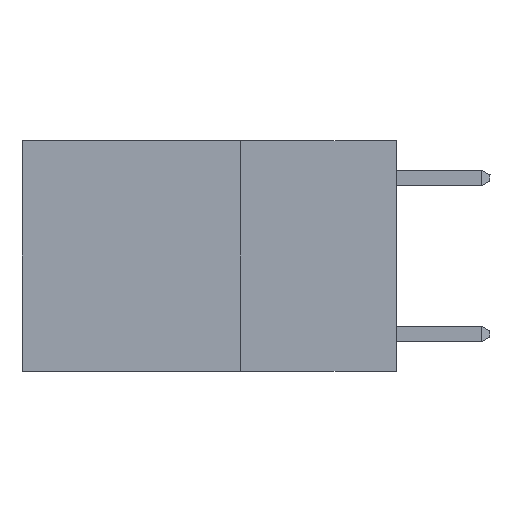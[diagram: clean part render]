
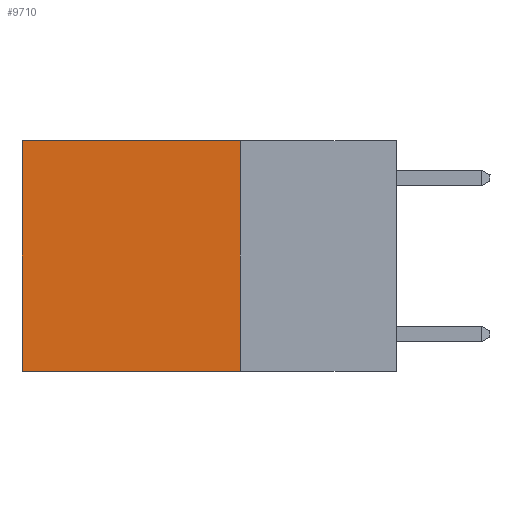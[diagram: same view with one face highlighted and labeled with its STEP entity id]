
A CAD part, left-side view. The second image highlights one B-rep face of the part: STEP entity #9710.
In plain terms, the highlighted planar face has unit normal (-1, 0, 0).
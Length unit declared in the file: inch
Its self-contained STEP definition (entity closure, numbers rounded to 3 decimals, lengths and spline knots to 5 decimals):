
#161 = DIRECTION ( 'NONE',  ( 0., 0., -1. ) ) ;
#735 = PLANE ( 'NONE',  #3707 ) ;
#923 = CARTESIAN_POINT ( 'NONE',  ( 0.2625, 0.6, 0. ) ) ;
#1424 = LINE ( 'NONE', #2410, #9687 ) ;
#2410 = CARTESIAN_POINT ( 'NONE',  ( 0.2625, 0.25, 0. ) ) ;
#3197 = CARTESIAN_POINT ( 'NONE',  ( 0.2625, 0.25, 0. ) ) ;
#3236 = DIRECTION ( 'NONE',  ( 1., 0., 0. ) ) ;
#3293 = ORIENTED_EDGE ( 'NONE', *, *, #4226, .F. ) ;
#3406 = EDGE_CURVE ( 'NONE', #9492, #10022, #1424, .T. ) ;
#3707 = AXIS2_PLACEMENT_3D ( 'NONE', #3197, #3236, #8784 ) ;
#4226 = EDGE_CURVE ( 'NONE', #9492, #7613, #9802, .T. ) ;
#4418 = VERTEX_POINT ( 'NONE', #7597 ) ;
#4994 = ORIENTED_EDGE ( 'NONE', *, *, #3406, .T. ) ;
#5407 = VECTOR ( 'NONE', #161, 39.37008 ) ;
#5448 = ORIENTED_EDGE ( 'NONE', *, *, #9461, .T. ) ;
#5813 = LINE ( 'NONE', #923, #7671 ) ;
#5844 = CARTESIAN_POINT ( 'NONE',  ( 0.2625, 0.25, 0. ) ) ;
#7046 = VECTOR ( 'NONE', #8673, 39.37008 ) ;
#7597 = CARTESIAN_POINT ( 'NONE',  ( 0.2625, 0.6, -0.37 ) ) ;
#7613 = VERTEX_POINT ( 'NONE', #8380 ) ;
#7671 = VECTOR ( 'NONE', #8949, 39.37008 ) ;
#7909 = CARTESIAN_POINT ( 'NONE',  ( 0.2625, 0.25, -0.37 ) ) ;
#8245 = CARTESIAN_POINT ( 'NONE',  ( 0.2625, 0.25, 0. ) ) ;
#8380 = CARTESIAN_POINT ( 'NONE',  ( 0.2625, 0.25, -0.37 ) ) ;
#8398 = FACE_OUTER_BOUND ( 'NONE', #9883, .T. ) ;
#8673 = DIRECTION ( 'NONE',  ( 0., 1., 0. ) ) ;
#8784 = DIRECTION ( 'NONE',  ( 0., 0., -1. ) ) ;
#8869 = LINE ( 'NONE', #7909, #7046 ) ;
#8872 = ORIENTED_EDGE ( 'NONE', *, *, #9996, .F. ) ;
#8949 = DIRECTION ( 'NONE',  ( 0., 0., -1. ) ) ;
#9461 = EDGE_CURVE ( 'NONE', #10022, #4418, #5813, .T. ) ;
#9492 = VERTEX_POINT ( 'NONE', #8245 ) ;
#9687 = VECTOR ( 'NONE', #10329, 39.37008 ) ;
#9710 = ADVANCED_FACE ( 'NONE', ( #8398 ), #735, .F. ) ;
#9802 = LINE ( 'NONE', #5844, #5407 ) ;
#9883 = EDGE_LOOP ( 'NONE', ( #5448, #8872, #3293, #4994 ) ) ;
#9996 = EDGE_CURVE ( 'NONE', #7613, #4418, #8869, .T. ) ;
#10022 = VERTEX_POINT ( 'NONE', #10295 ) ;
#10295 = CARTESIAN_POINT ( 'NONE',  ( 0.2625, 0.6, 0. ) ) ;
#10329 = DIRECTION ( 'NONE',  ( 0., 1., 0. ) ) ;
